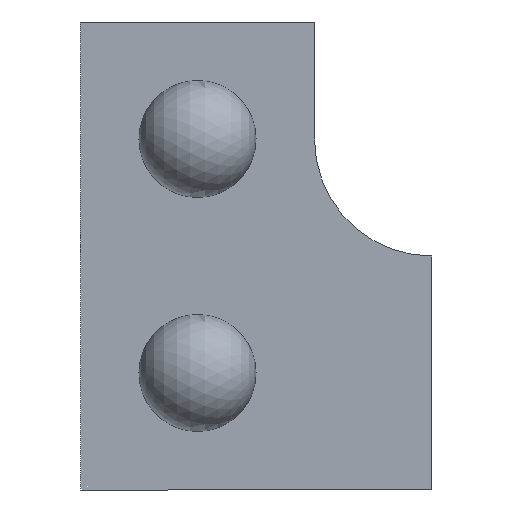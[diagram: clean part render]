
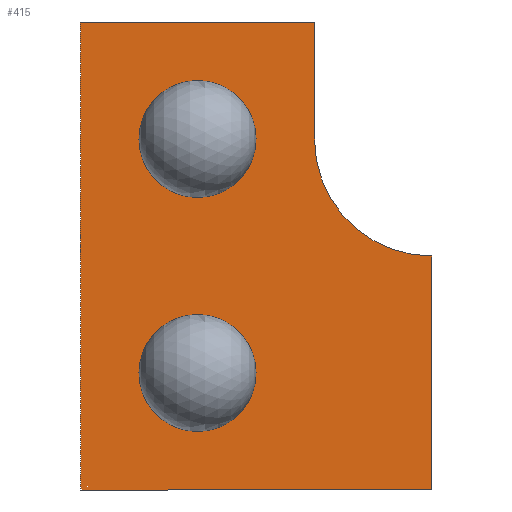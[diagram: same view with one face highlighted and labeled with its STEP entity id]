
A CAD part, left-side view. The second image highlights one B-rep face of the part: STEP entity #415.
In plain terms, the highlighted planar face has unit normal (-1, 0, 0).
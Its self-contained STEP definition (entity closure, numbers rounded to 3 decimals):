
#2 = LINE ( 'NONE', #90, #27 ) ;
#13 = ORIENTED_EDGE ( 'NONE', *, *, #89, .F. ) ;
#14 = CARTESIAN_POINT ( 'NONE',  ( 0., 0., 0. ) ) ;
#21 = EDGE_CURVE ( 'NONE', #267, #80, #221, .T. ) ;
#22 = EDGE_LOOP ( 'NONE', ( #98, #13, #239, #167, #202, #193 ) ) ;
#27 = VECTOR ( 'NONE', #309, 1000. ) ;
#28 = CIRCLE ( 'NONE', #254, 2.5 ) ;
#30 = ORIENTED_EDGE ( 'NONE', *, *, #21, .T. ) ;
#32 = DIRECTION ( 'NONE',  ( 1., 0., 0. ) ) ;
#44 = CARTESIAN_POINT ( 'NONE',  ( 0., 5., 0. ) ) ;
#47 = DIRECTION ( 'NONE',  ( 0., 0., -1. ) ) ;
#55 = VECTOR ( 'NONE', #95, 1000. ) ;
#57 = CARTESIAN_POINT ( 'NONE',  ( 0., 0., 5. ) ) ;
#61 = EDGE_LOOP ( 'NONE', ( #30, #115 ) ) ;
#80 = VERTEX_POINT ( 'NONE', #232 ) ;
#81 = DIRECTION ( 'NONE',  ( 0., 0., -1. ) ) ;
#85 = VERTEX_POINT ( 'NONE', #285 ) ;
#89 = EDGE_CURVE ( 'NONE', #399, #354, #282, .T. ) ;
#90 = CARTESIAN_POINT ( 'NONE',  ( 0., 20., 0. ) ) ;
#94 = CARTESIAN_POINT ( 'NONE',  ( 0., 15., -2.5 ) ) ;
#95 = DIRECTION ( 'NONE',  ( 0., 0., -1. ) ) ;
#97 = VERTEX_POINT ( 'NONE', #351 ) ;
#98 = ORIENTED_EDGE ( 'NONE', *, *, #326, .F. ) ;
#115 = ORIENTED_EDGE ( 'NONE', *, *, #419, .T. ) ;
#118 = VECTOR ( 'NONE', #313, 1000. ) ;
#147 = LINE ( 'NONE', #293, #236 ) ;
#149 = CARTESIAN_POINT ( 'NONE',  ( 0., 15., 0. ) ) ;
#161 = CARTESIAN_POINT ( 'NONE',  ( 0., 5., -15. ) ) ;
#163 = CARTESIAN_POINT ( 'NONE',  ( 0., 10., 5. ) ) ;
#166 = ORIENTED_EDGE ( 'NONE', *, *, #336, .T. ) ;
#167 = ORIENTED_EDGE ( 'NONE', *, *, #273, .T. ) ;
#169 = DIRECTION ( 'NONE',  ( 0., -1., 0. ) ) ;
#173 = AXIS2_PLACEMENT_3D ( 'NONE', #387, #200, #416 ) ;
#185 = VERTEX_POINT ( 'NONE', #332 ) ;
#190 = LINE ( 'NONE', #393, #258 ) ;
#191 = VERTEX_POINT ( 'NONE', #269 ) ;
#192 = CARTESIAN_POINT ( 'NONE',  ( 0., 15., -10. ) ) ;
#193 = ORIENTED_EDGE ( 'NONE', *, *, #377, .T. ) ;
#195 = CARTESIAN_POINT ( 'NONE',  ( 0., 10., 0. ) ) ;
#200 = DIRECTION ( 'NONE',  ( 1., 0., 0. ) ) ;
#202 = ORIENTED_EDGE ( 'NONE', *, *, #302, .T. ) ;
#208 = DIRECTION ( 'NONE',  ( 0., 0., 1. ) ) ;
#221 = CIRCLE ( 'NONE', #173, 2.5 ) ;
#231 = CARTESIAN_POINT ( 'NONE',  ( 0., 15., -10. ) ) ;
#232 = CARTESIAN_POINT ( 'NONE',  ( 0., 15., 2.5 ) ) ;
#234 = EDGE_CURVE ( 'NONE', #399, #191, #2, .T. ) ;
#236 = VECTOR ( 'NONE', #208, 1000. ) ;
#239 = ORIENTED_EDGE ( 'NONE', *, *, #234, .T. ) ;
#245 = EDGE_CURVE ( 'NONE', #185, #85, #390, .T. ) ;
#246 = DIRECTION ( 'NONE',  ( 1., 0., 0. ) ) ;
#250 = AXIS2_PLACEMENT_3D ( 'NONE', #14, #246, #47 ) ;
#254 = AXIS2_PLACEMENT_3D ( 'NONE', #149, #281, #349 ) ;
#257 = DIRECTION ( 'NONE',  ( 0., 0., -1. ) ) ;
#258 = VECTOR ( 'NONE', #169, 1000. ) ;
#267 = VERTEX_POINT ( 'NONE', #94 ) ;
#269 = CARTESIAN_POINT ( 'NONE',  ( 0., 20., -15. ) ) ;
#273 = EDGE_CURVE ( 'NONE', #191, #292, #190, .T. ) ;
#274 = DIRECTION ( 'NONE',  ( 1., 0., 0. ) ) ;
#276 = FACE_OUTER_BOUND ( 'NONE', #22, .T. ) ;
#281 = DIRECTION ( 'NONE',  ( 1., 0., 0. ) ) ;
#282 = LINE ( 'NONE', #57, #118 ) ;
#283 = AXIS2_PLACEMENT_3D ( 'NONE', #44, #274, #81 ) ;
#285 = CARTESIAN_POINT ( 'NONE',  ( 0., 15., -12.5 ) ) ;
#289 = CARTESIAN_POINT ( 'NONE',  ( 0., 10., 0. ) ) ;
#292 = VERTEX_POINT ( 'NONE', #161 ) ;
#293 = CARTESIAN_POINT ( 'NONE',  ( 0., 5., 0. ) ) ;
#296 = CIRCLE ( 'NONE', #283, 5. ) ;
#301 = CARTESIAN_POINT ( 'NONE',  ( 0., 20., 5. ) ) ;
#302 = EDGE_CURVE ( 'NONE', #292, #97, #147, .T. ) ;
#309 = DIRECTION ( 'NONE',  ( 0., 0., -1. ) ) ;
#313 = DIRECTION ( 'NONE',  ( 0., -1., 0. ) ) ;
#321 = DIRECTION ( 'NONE',  ( 0., 0., -1. ) ) ;
#326 = EDGE_CURVE ( 'NONE', #354, #378, #397, .T. ) ;
#331 = AXIS2_PLACEMENT_3D ( 'NONE', #231, #32, #257 ) ;
#332 = CARTESIAN_POINT ( 'NONE',  ( 0., 15., -7.5 ) ) ;
#336 = EDGE_CURVE ( 'NONE', #85, #185, #373, .T. ) ;
#338 = FACE_BOUND ( 'NONE', #400, .T. ) ;
#349 = DIRECTION ( 'NONE',  ( 0., 0., -1. ) ) ;
#351 = CARTESIAN_POINT ( 'NONE',  ( 0., 5., -5. ) ) ;
#354 = VERTEX_POINT ( 'NONE', #163 ) ;
#373 = CIRCLE ( 'NONE', #331, 2.5 ) ;
#377 = EDGE_CURVE ( 'NONE', #97, #378, #296, .T. ) ;
#378 = VERTEX_POINT ( 'NONE', #289 ) ;
#387 = CARTESIAN_POINT ( 'NONE',  ( 0., 15., 0. ) ) ;
#390 = CIRCLE ( 'NONE', #406, 2.5 ) ;
#393 = CARTESIAN_POINT ( 'NONE',  ( 0., 0., -15. ) ) ;
#397 = LINE ( 'NONE', #195, #55 ) ;
#399 = VERTEX_POINT ( 'NONE', #301 ) ;
#400 = EDGE_LOOP ( 'NONE', ( #166, #418 ) ) ;
#406 = AXIS2_PLACEMENT_3D ( 'NONE', #192, #410, #321 ) ;
#408 = PLANE ( 'NONE',  #250 ) ;
#410 = DIRECTION ( 'NONE',  ( 1., 0., 0. ) ) ;
#413 = FACE_BOUND ( 'NONE', #61, .T. ) ;
#415 = ADVANCED_FACE ( 'NONE', ( #338, #413, #276 ), #408, .F. ) ;
#416 = DIRECTION ( 'NONE',  ( 0., 0., -1. ) ) ;
#418 = ORIENTED_EDGE ( 'NONE', *, *, #245, .T. ) ;
#419 = EDGE_CURVE ( 'NONE', #80, #267, #28, .T. ) ;
